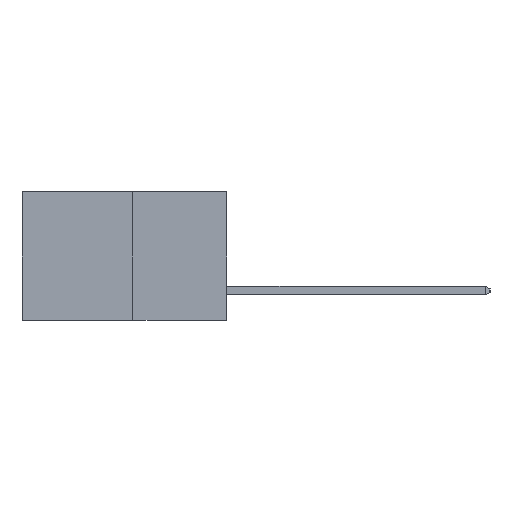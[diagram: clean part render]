
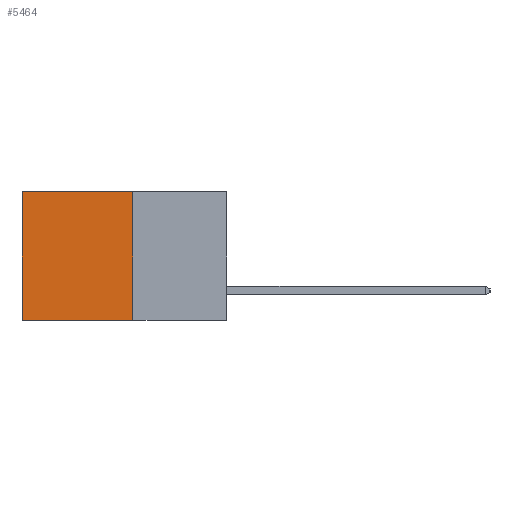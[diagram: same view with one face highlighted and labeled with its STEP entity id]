
A CAD part, left-side view. The second image highlights one B-rep face of the part: STEP entity #5464.
In plain terms, the highlighted planar face has unit normal (-1, 0, 0).
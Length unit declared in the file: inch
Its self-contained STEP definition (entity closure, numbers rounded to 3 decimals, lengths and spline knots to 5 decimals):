
#1845 = EDGE_CURVE ( 'NONE', #22569, #4402, #16843, .T. ) ;
#2371 = DIRECTION ( 'NONE',  ( 0., 1., 0. ) ) ;
#2599 = EDGE_CURVE ( 'NONE', #21918, #22569, #24162, .T. ) ;
#3138 = DIRECTION ( 'NONE',  ( 0., 0., -1. ) ) ;
#3164 = DIRECTION ( 'NONE',  ( 1., 0., 0. ) ) ;
#3457 = CARTESIAN_POINT ( 'NONE',  ( 0.277, 0.27, -0.37 ) ) ;
#3470 = CARTESIAN_POINT ( 'NONE',  ( 0.277, 0.27, -0.37 ) ) ;
#3686 = PLANE ( 'NONE',  #13862 ) ;
#3840 = FACE_OUTER_BOUND ( 'NONE', #5579, .T. ) ;
#4179 = ORIENTED_EDGE ( 'NONE', *, *, #22949, .T. ) ;
#4257 = EDGE_CURVE ( 'NONE', #8621, #4402, #11253, .T. ) ;
#4402 = VERTEX_POINT ( 'NONE', #24691 ) ;
#5464 = ADVANCED_FACE ( 'NONE', ( #3840 ), #3686, .F. ) ;
#5579 = EDGE_LOOP ( 'NONE', ( #15697, #24557, #8050, #4179 ) ) ;
#6589 = VECTOR ( 'NONE', #2371, 39.37008 ) ;
#7047 = CARTESIAN_POINT ( 'NONE',  ( 0.277, 0.59, 0. ) ) ;
#8050 = ORIENTED_EDGE ( 'NONE', *, *, #2599, .F. ) ;
#8621 = VERTEX_POINT ( 'NONE', #7047 ) ;
#9164 = CARTESIAN_POINT ( 'NONE',  ( 0.277, 0.59, -0.37 ) ) ;
#11085 = VECTOR ( 'NONE', #21317, 39.37008 ) ;
#11253 = LINE ( 'NONE', #9164, #15833 ) ;
#11540 = DIRECTION ( 'NONE',  ( 0., 0., -1. ) ) ;
#12365 = LINE ( 'NONE', #19768, #6589 ) ;
#13862 = AXIS2_PLACEMENT_3D ( 'NONE', #3457, #3164, #3138 ) ;
#14404 = CARTESIAN_POINT ( 'NONE',  ( 0.277, 0.27, -0.37 ) ) ;
#15697 = ORIENTED_EDGE ( 'NONE', *, *, #4257, .T. ) ;
#15833 = VECTOR ( 'NONE', #11540, 39.37008 ) ;
#16843 = LINE ( 'NONE', #3470, #11085 ) ;
#18018 = CARTESIAN_POINT ( 'NONE',  ( 0.277, 0.27, -0.37 ) ) ;
#18098 = DIRECTION ( 'NONE',  ( 0., 0., -1. ) ) ;
#19175 = VECTOR ( 'NONE', #18098, 39.37008 ) ;
#19768 = CARTESIAN_POINT ( 'NONE',  ( 0.277, 0.27, 0. ) ) ;
#21317 = DIRECTION ( 'NONE',  ( 0., 1., 0. ) ) ;
#21614 = CARTESIAN_POINT ( 'NONE',  ( 0.277, 0.27, 0. ) ) ;
#21918 = VERTEX_POINT ( 'NONE', #21614 ) ;
#22569 = VERTEX_POINT ( 'NONE', #14404 ) ;
#22949 = EDGE_CURVE ( 'NONE', #21918, #8621, #12365, .T. ) ;
#24162 = LINE ( 'NONE', #18018, #19175 ) ;
#24557 = ORIENTED_EDGE ( 'NONE', *, *, #1845, .F. ) ;
#24691 = CARTESIAN_POINT ( 'NONE',  ( 0.277, 0.59, -0.37 ) ) ;
